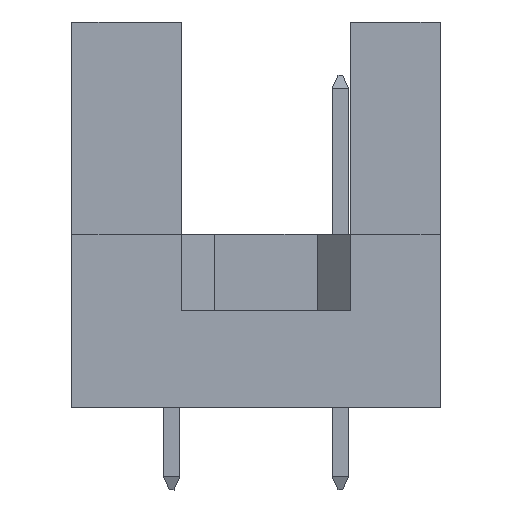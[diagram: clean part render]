
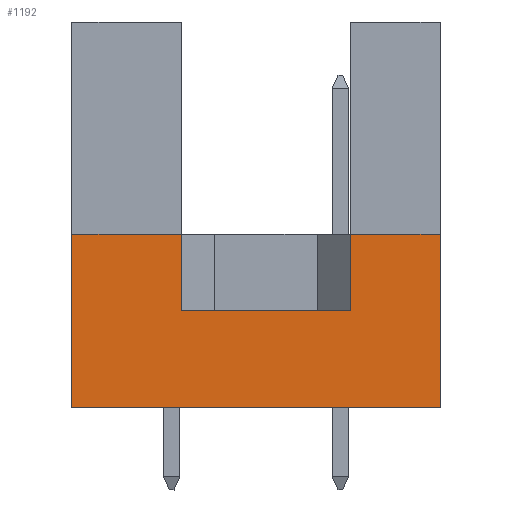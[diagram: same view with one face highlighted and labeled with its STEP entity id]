
A CAD part, left-side view. The second image highlights one B-rep face of the part: STEP entity #1192.
In plain terms, the highlighted planar face has unit normal (-1, 0, 0).
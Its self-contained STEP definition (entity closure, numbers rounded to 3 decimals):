
#4 = CARTESIAN_POINT ( 'NONE',  ( -19.9, 0., 0. ) ) ;
#5 = CARTESIAN_POINT ( 'NONE',  ( -19.9, 7.79, 5.2 ) ) ;
#68 = EDGE_CURVE ( 'NONE', #1815, #1257, #5613, .T. ) ;
#271 = ORIENTED_EDGE ( 'NONE', *, *, #1106, .F. ) ;
#357 = EDGE_CURVE ( 'NONE', #3634, #6105, #6334, .T. ) ;
#383 = CARTESIAN_POINT ( 'NONE',  ( -19.9, 11.1, 5.2 ) ) ;
#416 = VERTEX_POINT ( 'NONE', #2840 ) ;
#456 = VERTEX_POINT ( 'NONE', #4331 ) ;
#636 = ORIENTED_EDGE ( 'NONE', *, *, #3761, .T. ) ;
#748 = VERTEX_POINT ( 'NONE', #4 ) ;
#766 = DIRECTION ( 'NONE',  ( 0., 0., 1. ) ) ;
#777 = ORIENTED_EDGE ( 'NONE', *, *, #5046, .T. ) ;
#859 = CARTESIAN_POINT ( 'NONE',  ( -19.9, 0., 0. ) ) ;
#1097 = CARTESIAN_POINT ( 'NONE',  ( -19.9, 11.1, 0. ) ) ;
#1106 = EDGE_CURVE ( 'NONE', #416, #3634, #1918, .T. ) ;
#1136 = DIRECTION ( 'NONE',  ( 0., 0., -1. ) ) ;
#1192 = ADVANCED_FACE ( 'NONE', ( #4799 ), #2648, .F. ) ;
#1257 = VERTEX_POINT ( 'NONE', #3242 ) ;
#1352 = DIRECTION ( 'NONE',  ( 0., -1., 0. ) ) ;
#1480 = DIRECTION ( 'NONE',  ( 0., -1., 0. ) ) ;
#1775 = LINE ( 'NONE', #6671, #4330 ) ;
#1815 = VERTEX_POINT ( 'NONE', #4400 ) ;
#1918 = LINE ( 'NONE', #4092, #5696 ) ;
#2201 = CARTESIAN_POINT ( 'NONE',  ( -19.9, 7.79, 2.9 ) ) ;
#2441 = DIRECTION ( 'NONE',  ( 0., -1., 0. ) ) ;
#2515 = DIRECTION ( 'NONE',  ( 0., 0., 1. ) ) ;
#2648 = PLANE ( 'NONE',  #4675 ) ;
#2840 = CARTESIAN_POINT ( 'NONE',  ( -19.9, 2.71, 2.9 ) ) ;
#2893 = LINE ( 'NONE', #3390, #4216 ) ;
#2964 = ORIENTED_EDGE ( 'NONE', *, *, #4985, .F. ) ;
#2976 = ORIENTED_EDGE ( 'NONE', *, *, #6753, .F. ) ;
#3167 = LINE ( 'NONE', #2201, #5634 ) ;
#3209 = DIRECTION ( 'NONE',  ( 0., -1., 0. ) ) ;
#3242 = CARTESIAN_POINT ( 'NONE',  ( -19.9, 11.1, 5.2 ) ) ;
#3264 = CARTESIAN_POINT ( 'NONE',  ( -19.9, 2.71, 5.2 ) ) ;
#3390 = CARTESIAN_POINT ( 'NONE',  ( -19.9, 11.1, 0. ) ) ;
#3542 = DIRECTION ( 'NONE',  ( 0., 0., 1. ) ) ;
#3607 = VECTOR ( 'NONE', #3542, 1000. ) ;
#3634 = VERTEX_POINT ( 'NONE', #3264 ) ;
#3761 = EDGE_CURVE ( 'NONE', #748, #6105, #5601, .T. ) ;
#3874 = VECTOR ( 'NONE', #1480, 1000. ) ;
#4022 = DIRECTION ( 'NONE',  ( 0., 0., 1. ) ) ;
#4092 = CARTESIAN_POINT ( 'NONE',  ( -19.9, 2.71, 2.9 ) ) ;
#4216 = VECTOR ( 'NONE', #2441, 1000. ) ;
#4325 = VECTOR ( 'NONE', #766, 1000. ) ;
#4330 = VECTOR ( 'NONE', #1352, 1000. ) ;
#4331 = CARTESIAN_POINT ( 'NONE',  ( -19.9, 7.79, 2.9 ) ) ;
#4400 = CARTESIAN_POINT ( 'NONE',  ( -19.9, 11.1, 0. ) ) ;
#4639 = ORIENTED_EDGE ( 'NONE', *, *, #68, .F. ) ;
#4675 = AXIS2_PLACEMENT_3D ( 'NONE', #1097, #5336, #1136 ) ;
#4676 = ORIENTED_EDGE ( 'NONE', *, *, #6029, .T. ) ;
#4771 = CARTESIAN_POINT ( 'NONE',  ( -19.9, 0., 5.2 ) ) ;
#4799 = FACE_OUTER_BOUND ( 'NONE', #5478, .T. ) ;
#4985 = EDGE_CURVE ( 'NONE', #1257, #6277, #1775, .T. ) ;
#5034 = CARTESIAN_POINT ( 'NONE',  ( -19.9, 7.79, 2.9 ) ) ;
#5046 = EDGE_CURVE ( 'NONE', #1815, #748, #2893, .T. ) ;
#5073 = ORIENTED_EDGE ( 'NONE', *, *, #357, .F. ) ;
#5336 = DIRECTION ( 'NONE',  ( 1., 0., 0. ) ) ;
#5451 = VECTOR ( 'NONE', #2515, 1000. ) ;
#5478 = EDGE_LOOP ( 'NONE', ( #2976, #4676, #2964, #4639, #777, #636, #5073, #271 ) ) ;
#5601 = LINE ( 'NONE', #859, #5451 ) ;
#5613 = LINE ( 'NONE', #6807, #4325 ) ;
#5634 = VECTOR ( 'NONE', #3209, 1000. ) ;
#5696 = VECTOR ( 'NONE', #4022, 1000. ) ;
#6029 = EDGE_CURVE ( 'NONE', #456, #6277, #6826, .T. ) ;
#6105 = VERTEX_POINT ( 'NONE', #4771 ) ;
#6277 = VERTEX_POINT ( 'NONE', #5 ) ;
#6334 = LINE ( 'NONE', #383, #3874 ) ;
#6671 = CARTESIAN_POINT ( 'NONE',  ( -19.9, 11.1, 5.2 ) ) ;
#6753 = EDGE_CURVE ( 'NONE', #456, #416, #3167, .T. ) ;
#6807 = CARTESIAN_POINT ( 'NONE',  ( -19.9, 11.1, 0. ) ) ;
#6826 = LINE ( 'NONE', #5034, #3607 ) ;
